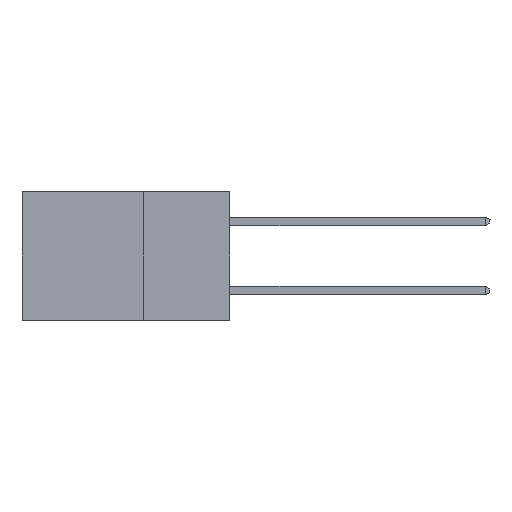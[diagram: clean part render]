
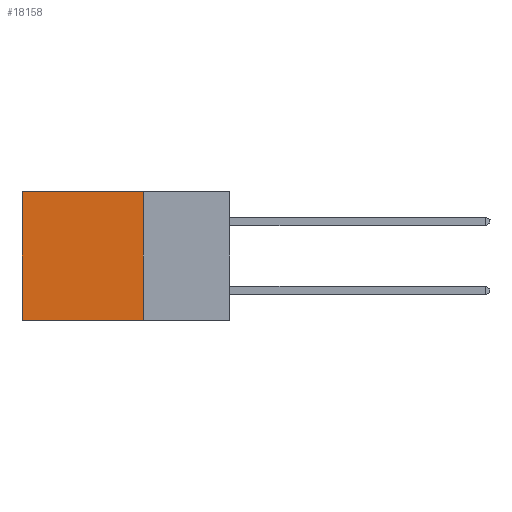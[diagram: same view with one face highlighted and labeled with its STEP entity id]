
A CAD part, left-side view. The second image highlights one B-rep face of the part: STEP entity #18158.
In plain terms, the highlighted planar face has unit normal (-1, 0, 0).
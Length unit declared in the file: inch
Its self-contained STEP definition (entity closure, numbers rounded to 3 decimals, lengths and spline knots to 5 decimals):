
#1216 = VECTOR ( 'NONE', #4266, 39.37008 ) ;
#1816 = CARTESIAN_POINT ( 'NONE',  ( 0.298, 0.25, 0. ) ) ;
#3323 = CARTESIAN_POINT ( 'NONE',  ( 0.298, 0.6, -0.37 ) ) ;
#4266 = DIRECTION ( 'NONE',  ( 0., 0., -1. ) ) ;
#5367 = VECTOR ( 'NONE', #28742, 39.37008 ) ;
#6477 = CARTESIAN_POINT ( 'NONE',  ( 0.298, 0.25, 0. ) ) ;
#6998 = AXIS2_PLACEMENT_3D ( 'NONE', #7047, #11974, #29108 ) ;
#7047 = CARTESIAN_POINT ( 'NONE',  ( 0.298, 0.25, 0. ) ) ;
#7744 = VECTOR ( 'NONE', #18731, 39.37008 ) ;
#8621 = VERTEX_POINT ( 'NONE', #3323 ) ;
#9423 = EDGE_CURVE ( 'NONE', #12840, #8621, #18023, .T. ) ;
#9526 = PLANE ( 'NONE',  #6998 ) ;
#11468 = VECTOR ( 'NONE', #18864, 39.37008 ) ;
#11911 = LINE ( 'NONE', #13965, #5367 ) ;
#11974 = DIRECTION ( 'NONE',  ( 1., 0., 0. ) ) ;
#12795 = FACE_OUTER_BOUND ( 'NONE', #23027, .T. ) ;
#12840 = VERTEX_POINT ( 'NONE', #20803 ) ;
#13965 = CARTESIAN_POINT ( 'NONE',  ( 0.298, 0.25, -0.37 ) ) ;
#14246 = LINE ( 'NONE', #1816, #1216 ) ;
#16717 = CARTESIAN_POINT ( 'NONE',  ( 0.298, 0.25, 0. ) ) ;
#18023 = LINE ( 'NONE', #21224, #11468 ) ;
#18158 = ADVANCED_FACE ( 'NONE', ( #12795 ), #9526, .F. ) ;
#18731 = DIRECTION ( 'NONE',  ( 0., 1., 0. ) ) ;
#18864 = DIRECTION ( 'NONE',  ( 0., 0., -1. ) ) ;
#19432 = EDGE_CURVE ( 'NONE', #22283, #21402, #14246, .T. ) ;
#19503 = ORIENTED_EDGE ( 'NONE', *, *, #26592, .T. ) ;
#20803 = CARTESIAN_POINT ( 'NONE',  ( 0.298, 0.6, 0. ) ) ;
#20973 = CARTESIAN_POINT ( 'NONE',  ( 0.298, 0.25, -0.37 ) ) ;
#21224 = CARTESIAN_POINT ( 'NONE',  ( 0.298, 0.6, 0. ) ) ;
#21402 = VERTEX_POINT ( 'NONE', #20973 ) ;
#21509 = EDGE_CURVE ( 'NONE', #21402, #8621, #11911, .T. ) ;
#22283 = VERTEX_POINT ( 'NONE', #16717 ) ;
#23027 = EDGE_LOOP ( 'NONE', ( #29995, #28401, #30674, #19503 ) ) ;
#26592 = EDGE_CURVE ( 'NONE', #22283, #12840, #27343, .T. ) ;
#27343 = LINE ( 'NONE', #6477, #7744 ) ;
#28401 = ORIENTED_EDGE ( 'NONE', *, *, #21509, .F. ) ;
#28742 = DIRECTION ( 'NONE',  ( 0., 1., 0. ) ) ;
#29108 = DIRECTION ( 'NONE',  ( 0., 0., -1. ) ) ;
#29995 = ORIENTED_EDGE ( 'NONE', *, *, #9423, .T. ) ;
#30674 = ORIENTED_EDGE ( 'NONE', *, *, #19432, .F. ) ;
